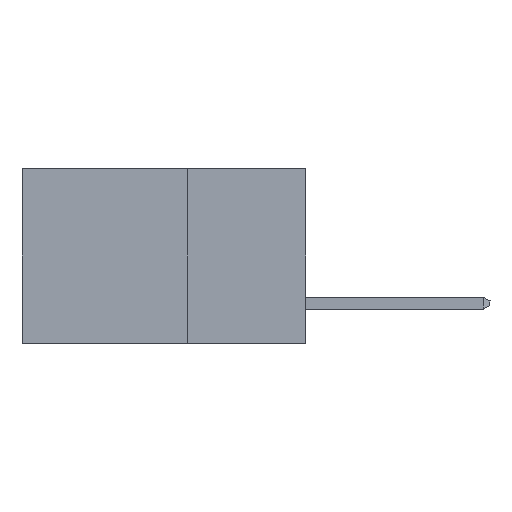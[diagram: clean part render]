
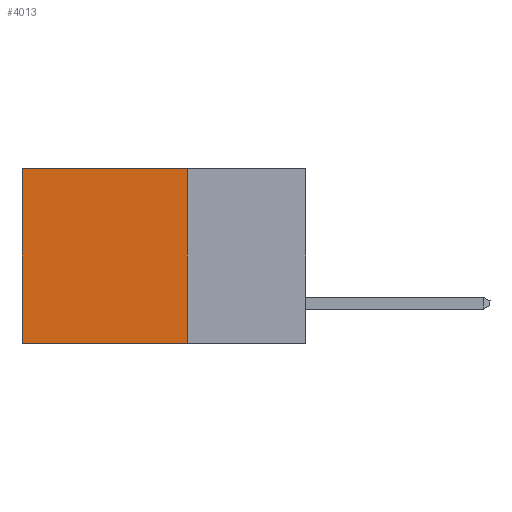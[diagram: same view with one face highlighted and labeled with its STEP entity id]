
A CAD part, left-side view. The second image highlights one B-rep face of the part: STEP entity #4013.
In plain terms, the highlighted planar face has unit normal (-1, 0, 0).
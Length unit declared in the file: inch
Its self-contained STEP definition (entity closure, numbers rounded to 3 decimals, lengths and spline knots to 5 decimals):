
#156 = EDGE_CURVE ( 'NONE', #10486, #13204, #2670, .T. ) ;
#817 = DIRECTION ( 'NONE',  ( 1., 0., 0. ) ) ;
#826 = DIRECTION ( 'NONE',  ( 0., 1., 0. ) ) ;
#1478 = VERTEX_POINT ( 'NONE', #13158 ) ;
#2145 = CARTESIAN_POINT ( 'NONE',  ( 0.298, 0.25, 0. ) ) ;
#2670 = LINE ( 'NONE', #6660, #5084 ) ;
#3656 = EDGE_CURVE ( 'NONE', #1478, #10486, #8177, .T. ) ;
#3765 = DIRECTION ( 'NONE',  ( 0., 1., 0. ) ) ;
#4013 = ADVANCED_FACE ( 'NONE', ( #6558 ), #14914, .F. ) ;
#4462 = ORIENTED_EDGE ( 'NONE', *, *, #6457, .F. ) ;
#4662 = VERTEX_POINT ( 'NONE', #8153 ) ;
#5018 = CARTESIAN_POINT ( 'NONE',  ( 0.298, 0.6, 0. ) ) ;
#5084 = VECTOR ( 'NONE', #11217, 39.37008 ) ;
#6457 = EDGE_CURVE ( 'NONE', #4662, #13204, #10502, .T. ) ;
#6558 = FACE_OUTER_BOUND ( 'NONE', #12590, .T. ) ;
#6660 = CARTESIAN_POINT ( 'NONE',  ( 0.298, 0.6, 0. ) ) ;
#7126 = DIRECTION ( 'NONE',  ( 0., 0., -1. ) ) ;
#7866 = CARTESIAN_POINT ( 'NONE',  ( 0.298, 0.25, 0. ) ) ;
#8142 = EDGE_CURVE ( 'NONE', #1478, #4662, #11377, .T. ) ;
#8153 = CARTESIAN_POINT ( 'NONE',  ( 0.298, 0.25, -0.37 ) ) ;
#8177 = LINE ( 'NONE', #10691, #8703 ) ;
#8432 = ORIENTED_EDGE ( 'NONE', *, *, #8142, .F. ) ;
#8703 = VECTOR ( 'NONE', #3765, 39.37008 ) ;
#9672 = ORIENTED_EDGE ( 'NONE', *, *, #156, .T. ) ;
#10486 = VERTEX_POINT ( 'NONE', #5018 ) ;
#10502 = LINE ( 'NONE', #13812, #13279 ) ;
#10691 = CARTESIAN_POINT ( 'NONE',  ( 0.298, 0.25, 0. ) ) ;
#11217 = DIRECTION ( 'NONE',  ( 0., 0., -1. ) ) ;
#11307 = AXIS2_PLACEMENT_3D ( 'NONE', #7866, #817, #7126 ) ;
#11377 = LINE ( 'NONE', #2145, #12675 ) ;
#12590 = EDGE_LOOP ( 'NONE', ( #9672, #4462, #8432, #15200 ) ) ;
#12675 = VECTOR ( 'NONE', #13917, 39.37008 ) ;
#13158 = CARTESIAN_POINT ( 'NONE',  ( 0.298, 0.25, 0. ) ) ;
#13204 = VERTEX_POINT ( 'NONE', #13723 ) ;
#13279 = VECTOR ( 'NONE', #826, 39.37008 ) ;
#13723 = CARTESIAN_POINT ( 'NONE',  ( 0.298, 0.6, -0.37 ) ) ;
#13812 = CARTESIAN_POINT ( 'NONE',  ( 0.298, 0.25, -0.37 ) ) ;
#13917 = DIRECTION ( 'NONE',  ( 0., 0., -1. ) ) ;
#14914 = PLANE ( 'NONE',  #11307 ) ;
#15200 = ORIENTED_EDGE ( 'NONE', *, *, #3656, .T. ) ;
